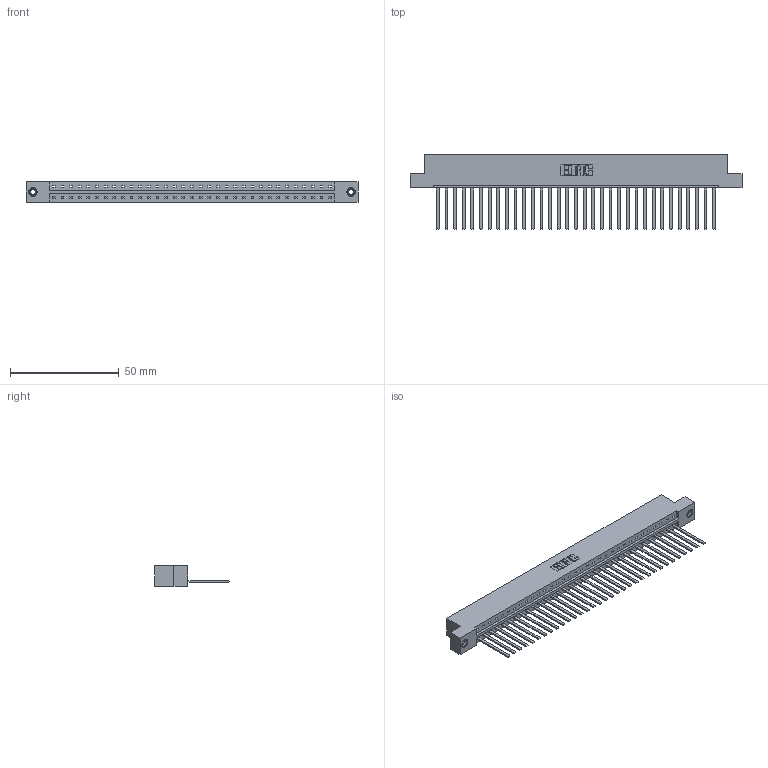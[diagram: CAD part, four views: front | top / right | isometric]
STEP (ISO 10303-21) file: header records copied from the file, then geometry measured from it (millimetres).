
FILE_DESCRIPTION (( 'STEP AP203' ), '1' );
FILE_NAME ('833-033-544-108.STEP', '2020-06-02T20:36:57', ( '' ), ( '' ), 'SwSTEP 2.0', 'SolidWorks 2020', '' );
FILE_SCHEMA (( 'CONFIG_CONTROL_DESIGN' ));
Length unit declared in the file: inch
Products named in the file (4): 345-292-001_345-293-144; 833 Part_Flush - .156 Dia - TI; 345-250-001_345-250-003-102; 833-033-544-108
Assembly tree (36 placements, depth 2):
  833-033-544-108
    833 Part_Flush - .156 Dia - TI
    345-292-001_345-293-144  x33
    345-250-001_345-250-003-102  x2
Bounding box: 152.3 x 34.3 x 9.4 mm (x, y, z)
Volume: 15623.8 mm3; surface area: 18114.3 mm2
Topology: 36 solids, 36 shells, 1890 faces, 5661 edges, 3722 vertices
Faces by surface type: plane 1356, cylinder 518, cone 12, torus 4
Entity records: 22340 total; most frequent: CARTESIAN_POINT 3836, ORIENTED_EDGE 3798, DIRECTION 3283, EDGE_CURVE 1899, LINE 1755, VECTOR 1755, VERTEX_POINT 1260, AXIS2_PLACEMENT_3D 764
